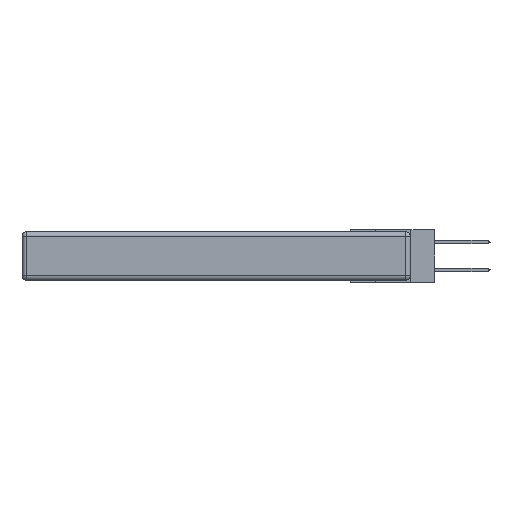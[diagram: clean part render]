
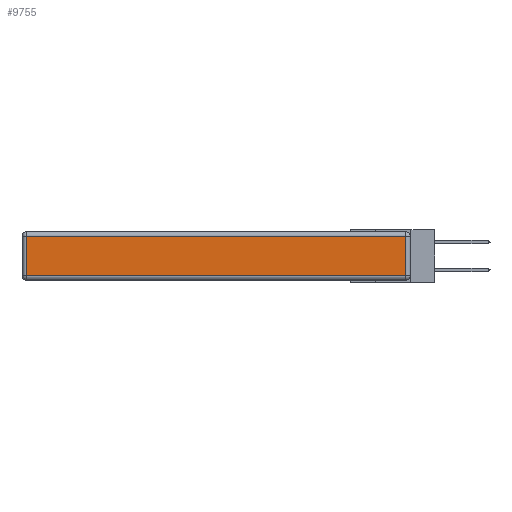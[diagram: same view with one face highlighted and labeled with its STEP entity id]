
A CAD part, left-side view. The second image highlights one B-rep face of the part: STEP entity #9755.
In plain terms, the highlighted planar face has unit normal (-1, 0, 0).
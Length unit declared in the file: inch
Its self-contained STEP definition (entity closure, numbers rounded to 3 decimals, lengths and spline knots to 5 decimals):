
#323 = CARTESIAN_POINT ( 'NONE',  ( 0., 2.72, -0.313 ) ) ;
#459 = VECTOR ( 'NONE', #1229, 39.37008 ) ;
#716 = EDGE_CURVE ( 'NONE', #14412, #16063, #19196, .T. ) ;
#849 = CARTESIAN_POINT ( 'NONE',  ( 0., 0.03, -0.343 ) ) ;
#1091 = VECTOR ( 'NONE', #15637, 39.37008 ) ;
#1229 = DIRECTION ( 'NONE',  ( 0., 1., 0. ) ) ;
#2734 = AXIS2_PLACEMENT_3D ( 'NONE', #14924, #5108, #13348 ) ;
#2790 = EDGE_CURVE ( 'NONE', #12910, #14412, #8034, .T. ) ;
#2940 = ORIENTED_EDGE ( 'NONE', *, *, #716, .T. ) ;
#4032 = VECTOR ( 'NONE', #8580, 39.37008 ) ;
#4214 = EDGE_CURVE ( 'NONE', #5010, #12910, #13594, .T. ) ;
#4306 = ORIENTED_EDGE ( 'NONE', *, *, #4214, .T. ) ;
#4443 = ORIENTED_EDGE ( 'NONE', *, *, #2790, .T. ) ;
#4808 = DIRECTION ( 'NONE',  ( 0., -1., 0. ) ) ;
#5010 = VERTEX_POINT ( 'NONE', #323 ) ;
#5108 = DIRECTION ( 'NONE',  ( -1., 0., 0. ) ) ;
#7989 = FACE_OUTER_BOUND ( 'NONE', #12640, .T. ) ;
#8034 = LINE ( 'NONE', #849, #1091 ) ;
#8538 = PLANE ( 'NONE',  #2734 ) ;
#8580 = DIRECTION ( 'NONE',  ( 0., 0., -1. ) ) ;
#9755 = ADVANCED_FACE ( 'NONE', ( #7989 ), #8538, .T. ) ;
#11718 = CARTESIAN_POINT ( 'NONE',  ( 0., 2.72, -0.03 ) ) ;
#12069 = EDGE_CURVE ( 'NONE', #16063, #5010, #16345, .T. ) ;
#12640 = EDGE_LOOP ( 'NONE', ( #4306, #4443, #2940, #19570 ) ) ;
#12910 = VERTEX_POINT ( 'NONE', #13502 ) ;
#13176 = VECTOR ( 'NONE', #4808, 39.37008 ) ;
#13348 = DIRECTION ( 'NONE',  ( 0., 0., 1. ) ) ;
#13502 = CARTESIAN_POINT ( 'NONE',  ( 0., 0.03, -0.313 ) ) ;
#13594 = LINE ( 'NONE', #16149, #13176 ) ;
#13666 = CARTESIAN_POINT ( 'NONE',  ( 0., 2.72, -0.343 ) ) ;
#14281 = CARTESIAN_POINT ( 'NONE',  ( 0., 2.75, -0.03 ) ) ;
#14412 = VERTEX_POINT ( 'NONE', #16967 ) ;
#14924 = CARTESIAN_POINT ( 'NONE',  ( 0., 0., -0.343 ) ) ;
#15637 = DIRECTION ( 'NONE',  ( 0., 0., 1. ) ) ;
#16063 = VERTEX_POINT ( 'NONE', #11718 ) ;
#16149 = CARTESIAN_POINT ( 'NONE',  ( 0., 0., -0.313 ) ) ;
#16345 = LINE ( 'NONE', #13666, #4032 ) ;
#16967 = CARTESIAN_POINT ( 'NONE',  ( 0., 0.03, -0.03 ) ) ;
#19196 = LINE ( 'NONE', #14281, #459 ) ;
#19570 = ORIENTED_EDGE ( 'NONE', *, *, #12069, .T. ) ;
